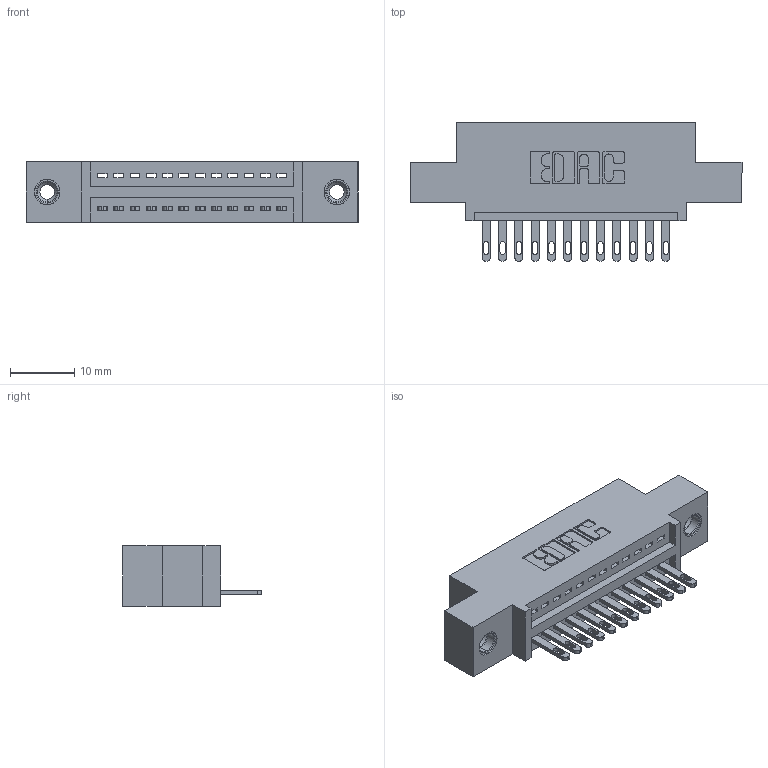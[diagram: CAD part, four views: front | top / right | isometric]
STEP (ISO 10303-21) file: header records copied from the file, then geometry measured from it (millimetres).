
FILE_DESCRIPTION (( 'STEP AP203' ), '1' );
FILE_NAME ('895-012-500-408.STEP', '2020-09-25T01:20:48', ( '' ), ( '' ), 'SwSTEP 2.0', 'SolidWorks 2020', '' );
FILE_SCHEMA (( 'CONFIG_CONTROL_DESIGN' ));
Length unit declared in the file: inch
Products named in the file (4): 345-250-001_345-250-003-102; 845 Part_0.110 Offset - 0.156 Dia-TI; 345-292-001_345-293-100; 895-012-500-408
Assembly tree (15 placements, depth 2):
  895-012-500-408
    845 Part_0.110 Offset - 0.156 Dia-TI
    345-292-001_345-293-100  x12
    345-250-001_345-250-003-102  x2
Bounding box: 51.69 x 21.51 x 9.4 mm (x, y, z)
Volume: 4591.3 mm3; surface area: 5821.6 mm2
Topology: 15 solids, 15 shells, 838 faces, 2505 edges, 1662 vertices
Faces by surface type: plane 524, cylinder 298, cone 12, torus 4
Entity records: 14318 total; most frequent: CARTESIAN_POINT 2463, ORIENTED_EDGE 2402, DIRECTION 2223, EDGE_CURVE 1201, VECTOR 997, LINE 997, VERTEX_POINT 796, AXIS2_PLACEMENT_3D 613
